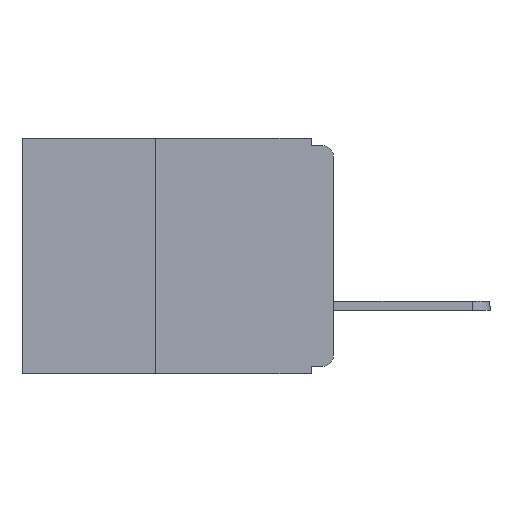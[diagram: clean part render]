
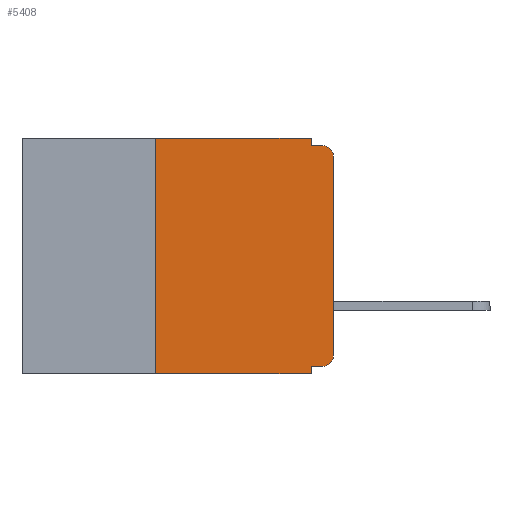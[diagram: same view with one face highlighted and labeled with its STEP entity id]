
A CAD part, left-side view. The second image highlights one B-rep face of the part: STEP entity #5408.
In plain terms, the highlighted planar face has unit normal (-1, 0, 0).
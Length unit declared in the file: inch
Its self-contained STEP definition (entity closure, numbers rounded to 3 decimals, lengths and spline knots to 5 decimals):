
#258 = DIRECTION ( 'NONE',  ( 0., 0., 1. ) ) ;
#891 = EDGE_CURVE ( 'NONE', #17725, #12135, #3360, .T. ) ;
#1163 = ORIENTED_EDGE ( 'NONE', *, *, #12938, .F. ) ;
#1240 = EDGE_CURVE ( 'NONE', #12135, #13770, #19030, .T. ) ;
#1273 = DIRECTION ( 'NONE',  ( 0., -1., 0. ) ) ;
#1722 = VECTOR ( 'NONE', #258, 39.37008 ) ;
#1838 = CARTESIAN_POINT ( 'NONE',  ( 0., 0., -0.32 ) ) ;
#1925 = CARTESIAN_POINT ( 'NONE',  ( 0., 0.031, -0.01 ) ) ;
#1942 = ORIENTED_EDGE ( 'NONE', *, *, #14693, .F. ) ;
#2040 = CARTESIAN_POINT ( 'NONE',  ( 0., 0.25, -0.33 ) ) ;
#2046 = VERTEX_POINT ( 'NONE', #21897 ) ;
#2048 = VECTOR ( 'NONE', #3612, 39.37008 ) ;
#2275 = VECTOR ( 'NONE', #1273, 39.37008 ) ;
#2277 = DIRECTION ( 'NONE',  ( 0., 0., -1. ) ) ;
#2503 = VERTEX_POINT ( 'NONE', #22589 ) ;
#2763 = ORIENTED_EDGE ( 'NONE', *, *, #5787, .F. ) ;
#2873 = VECTOR ( 'NONE', #16304, 39.37008 ) ;
#3360 = CIRCLE ( 'NONE', #8746, 0.015 ) ;
#3483 = CARTESIAN_POINT ( 'NONE',  ( 0., 0.015, -0.025 ) ) ;
#3612 = DIRECTION ( 'NONE',  ( 0., 1., 0. ) ) ;
#4180 = ORIENTED_EDGE ( 'NONE', *, *, #4968, .T. ) ;
#4327 = DIRECTION ( 'NONE',  ( 0., 0., 1. ) ) ;
#4755 = CARTESIAN_POINT ( 'NONE',  ( 0., 0.437, 0. ) ) ;
#4790 = VERTEX_POINT ( 'NONE', #1925 ) ;
#4968 = EDGE_CURVE ( 'NONE', #13616, #16707, #15367, .T. ) ;
#5209 = DIRECTION ( 'NONE',  ( 0., -1., 0. ) ) ;
#5236 = CARTESIAN_POINT ( 'NONE',  ( 0., 0.437, -0.33 ) ) ;
#5248 = AXIS2_PLACEMENT_3D ( 'NONE', #4755, #6546, #18809 ) ;
#5296 = DIRECTION ( 'NONE',  ( 0., 0., -1. ) ) ;
#5408 = ADVANCED_FACE ( 'NONE', ( #6542 ), #15315, .F. ) ;
#5590 = ORIENTED_EDGE ( 'NONE', *, *, #5605, .F. ) ;
#5605 = EDGE_CURVE ( 'NONE', #19515, #2503, #7344, .T. ) ;
#5787 = EDGE_CURVE ( 'NONE', #2503, #4790, #16978, .T. ) ;
#6416 = EDGE_CURVE ( 'NONE', #20790, #16707, #21759, .T. ) ;
#6542 = FACE_OUTER_BOUND ( 'NONE', #20702, .T. ) ;
#6546 = DIRECTION ( 'NONE',  ( 1., 0., 0. ) ) ;
#6685 = EDGE_CURVE ( 'NONE', #4790, #2046, #16399, .T. ) ;
#6795 = LINE ( 'NONE', #1838, #2048 ) ;
#6941 = AXIS2_PLACEMENT_3D ( 'NONE', #3483, #15857, #5296 ) ;
#7344 = LINE ( 'NONE', #15850, #20188 ) ;
#7536 = ORIENTED_EDGE ( 'NONE', *, *, #6416, .F. ) ;
#8409 = CARTESIAN_POINT ( 'NONE',  ( 0., 0.031, -0.33 ) ) ;
#8557 = DIRECTION ( 'NONE',  ( 0., 0., -1. ) ) ;
#8593 = ORIENTED_EDGE ( 'NONE', *, *, #6685, .F. ) ;
#8746 = AXIS2_PLACEMENT_3D ( 'NONE', #9655, #9857, #8557 ) ;
#9369 = CARTESIAN_POINT ( 'NONE',  ( 0., 0.25, 0. ) ) ;
#9655 = CARTESIAN_POINT ( 'NONE',  ( 0., 0.015, -0.305 ) ) ;
#9705 = CARTESIAN_POINT ( 'NONE',  ( 0., 0.25, -0.33 ) ) ;
#9752 = EDGE_CURVE ( 'NONE', #13770, #2046, #21177, .T. ) ;
#9857 = DIRECTION ( 'NONE',  ( -1., 0., 0. ) ) ;
#10169 = CARTESIAN_POINT ( 'NONE',  ( 0., 0., -0.025 ) ) ;
#10694 = VECTOR ( 'NONE', #20988, 39.37008 ) ;
#12135 = VERTEX_POINT ( 'NONE', #18665 ) ;
#12877 = CARTESIAN_POINT ( 'NONE',  ( 0., 0.031, -0.33 ) ) ;
#12938 = EDGE_CURVE ( 'NONE', #17725, #20790, #6795, .T. ) ;
#13497 = ORIENTED_EDGE ( 'NONE', *, *, #9752, .T. ) ;
#13616 = VERTEX_POINT ( 'NONE', #9705 ) ;
#13770 = VERTEX_POINT ( 'NONE', #10169 ) ;
#14435 = VECTOR ( 'NONE', #4327, 39.37008 ) ;
#14541 = CARTESIAN_POINT ( 'NONE',  ( 0., 0.031, 0. ) ) ;
#14693 = EDGE_CURVE ( 'NONE', #13616, #19515, #20411, .T. ) ;
#15169 = CARTESIAN_POINT ( 'NONE',  ( 0., 0.031, -0.32 ) ) ;
#15315 = PLANE ( 'NONE',  #5248 ) ;
#15367 = LINE ( 'NONE', #5236, #10694 ) ;
#15850 = CARTESIAN_POINT ( 'NONE',  ( 0., 0.437, 0. ) ) ;
#15857 = DIRECTION ( 'NONE',  ( -1., 0., 0. ) ) ;
#16304 = DIRECTION ( 'NONE',  ( 0., 0., -1. ) ) ;
#16399 = LINE ( 'NONE', #20542, #2275 ) ;
#16707 = VERTEX_POINT ( 'NONE', #8409 ) ;
#16978 = LINE ( 'NONE', #14541, #2873 ) ;
#17428 = CARTESIAN_POINT ( 'NONE',  ( 0., 0., 0. ) ) ;
#17725 = VERTEX_POINT ( 'NONE', #18249 ) ;
#18249 = CARTESIAN_POINT ( 'NONE',  ( 0., 0.015, -0.32 ) ) ;
#18557 = ORIENTED_EDGE ( 'NONE', *, *, #891, .T. ) ;
#18665 = CARTESIAN_POINT ( 'NONE',  ( 0., 0., -0.305 ) ) ;
#18809 = DIRECTION ( 'NONE',  ( 0., 0., -1. ) ) ;
#19030 = LINE ( 'NONE', #17428, #14435 ) ;
#19515 = VERTEX_POINT ( 'NONE', #9369 ) ;
#20188 = VECTOR ( 'NONE', #5209, 39.37008 ) ;
#20411 = LINE ( 'NONE', #2040, #1722 ) ;
#20542 = CARTESIAN_POINT ( 'NONE',  ( 0., 0., -0.01 ) ) ;
#20702 = EDGE_LOOP ( 'NONE', ( #21838, #13497, #8593, #2763, #5590, #1942, #4180, #7536, #1163, #18557 ) ) ;
#20790 = VERTEX_POINT ( 'NONE', #15169 ) ;
#20988 = DIRECTION ( 'NONE',  ( 0., -1., 0. ) ) ;
#21177 = CIRCLE ( 'NONE', #6941, 0.015 ) ;
#21759 = LINE ( 'NONE', #12877, #22312 ) ;
#21838 = ORIENTED_EDGE ( 'NONE', *, *, #1240, .T. ) ;
#21897 = CARTESIAN_POINT ( 'NONE',  ( 0., 0.015, -0.01 ) ) ;
#22312 = VECTOR ( 'NONE', #2277, 39.37008 ) ;
#22589 = CARTESIAN_POINT ( 'NONE',  ( 0., 0.031, 0. ) ) ;
